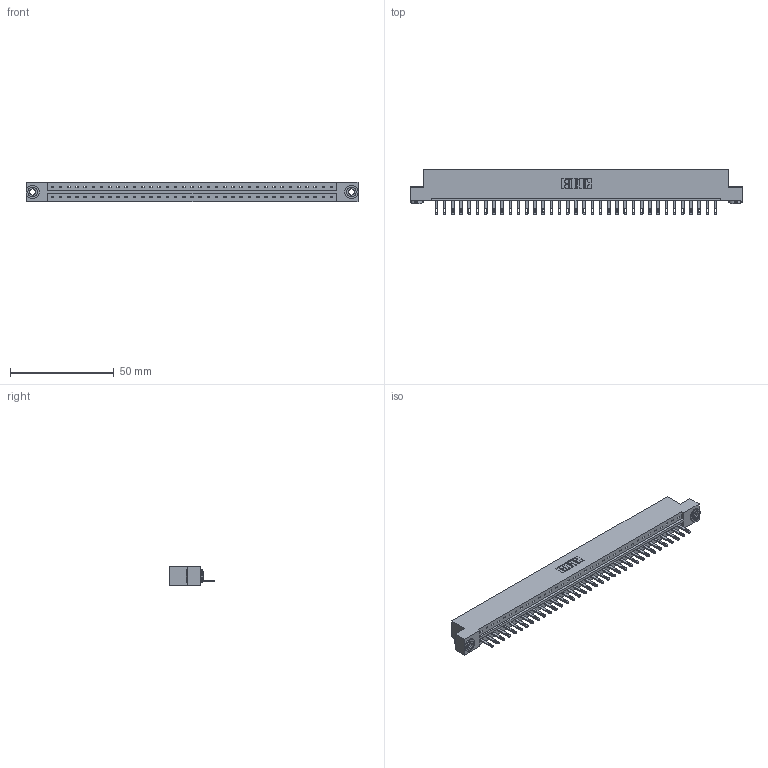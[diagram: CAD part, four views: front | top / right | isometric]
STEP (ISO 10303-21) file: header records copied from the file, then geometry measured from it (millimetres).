
FILE_DESCRIPTION (( 'STEP AP203' ), '1' );
FILE_NAME ('833-035-500-103.STEP', '2020-06-02T23:56:51', ( '' ), ( '' ), 'SwSTEP 2.0', 'SolidWorks 2020', '' );
FILE_SCHEMA (( 'CONFIG_CONTROL_DESIGN' ));
Length unit declared in the file: inch
Products named in the file (4): 833 Part_Flush - .156 Dia - TH; 345-250-002_345-250-002-102; 345-292-001_345-293-100; 833-035-500-103
Assembly tree (38 placements, depth 2):
  833-035-500-103
    833 Part_Flush - .156 Dia - TH
    345-292-001_345-293-100  x35
    345-250-002_345-250-002-102  x2
Bounding box: 160.22 x 21.85 x 9.4 mm (x, y, z)
Volume: 16103.8 mm3; surface area: 17690.9 mm2
Topology: 38 solids, 38 shells, 2042 faces, 6267 edges, 4174 vertices
Faces by surface type: plane 1340, cylinder 694, cone 8
Entity records: 22882 total; most frequent: CARTESIAN_POINT 3926, ORIENTED_EDGE 3890, DIRECTION 3361, EDGE_CURVE 1945, VECTOR 1789, LINE 1789, VERTEX_POINT 1294, AXIS2_PLACEMENT_3D 786
